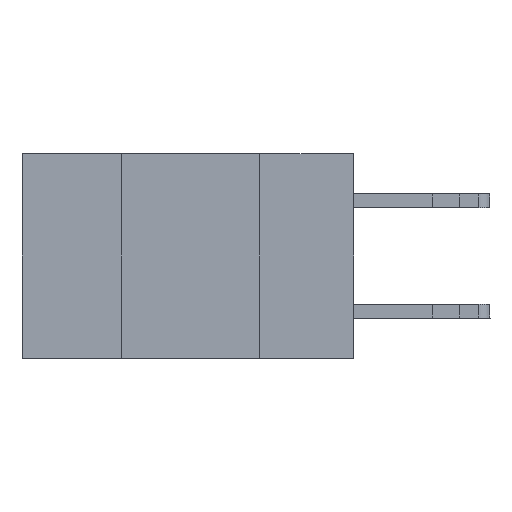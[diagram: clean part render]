
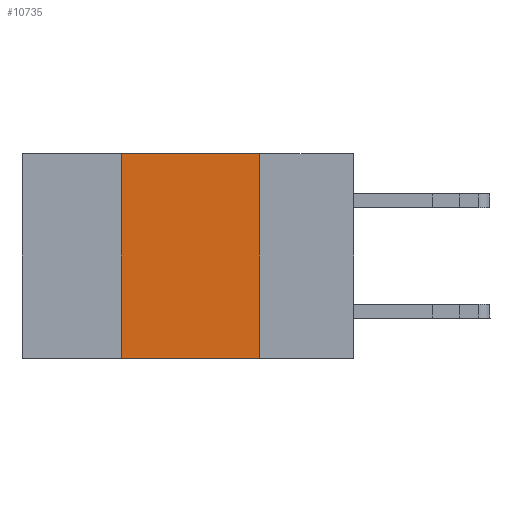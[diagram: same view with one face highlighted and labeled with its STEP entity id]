
A CAD part, left-side view. The second image highlights one B-rep face of the part: STEP entity #10735.
In plain terms, the highlighted planar face has unit normal (-1, 0, 0).
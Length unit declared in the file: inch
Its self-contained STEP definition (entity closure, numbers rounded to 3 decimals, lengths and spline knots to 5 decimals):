
#578 = EDGE_CURVE ( 'NONE', #19235, #1593, #18626, .T. ) ;
#873 = LINE ( 'NONE', #1668, #14500 ) ;
#1593 = VERTEX_POINT ( 'NONE', #20827 ) ;
#1668 = CARTESIAN_POINT ( 'NONE',  ( 0., 0.17, 0. ) ) ;
#1805 = FACE_OUTER_BOUND ( 'NONE', #4967, .T. ) ;
#2194 = DIRECTION ( 'NONE',  ( 0., -1., 0. ) ) ;
#3509 = LINE ( 'NONE', #20020, #16504 ) ;
#4251 = CARTESIAN_POINT ( 'NONE',  ( 0., 0.42, -0.37 ) ) ;
#4628 = DIRECTION ( 'NONE',  ( 0., 0., 1. ) ) ;
#4967 = EDGE_LOOP ( 'NONE', ( #20766, #8274, #18511, #7279 ) ) ;
#5052 = DIRECTION ( 'NONE',  ( 0., 0., -1. ) ) ;
#5714 = VECTOR ( 'NONE', #4628, 39.37008 ) ;
#7279 = ORIENTED_EDGE ( 'NONE', *, *, #16860, .T. ) ;
#8274 = ORIENTED_EDGE ( 'NONE', *, *, #10631, .F. ) ;
#8470 = DIRECTION ( 'NONE',  ( 0., 0., -1. ) ) ;
#9237 = CARTESIAN_POINT ( 'NONE',  ( 0., 0.6, 0. ) ) ;
#10277 = AXIS2_PLACEMENT_3D ( 'NONE', #9237, #15205, #5052 ) ;
#10631 = EDGE_CURVE ( 'NONE', #1593, #13225, #21349, .T. ) ;
#10735 = ADVANCED_FACE ( 'NONE', ( #1805 ), #17678, .F. ) ;
#11419 = CARTESIAN_POINT ( 'NONE',  ( 0., 0.17, -0.37 ) ) ;
#13225 = VERTEX_POINT ( 'NONE', #18328 ) ;
#14500 = VECTOR ( 'NONE', #8470, 39.37008 ) ;
#14962 = VERTEX_POINT ( 'NONE', #11419 ) ;
#15157 = DIRECTION ( 'NONE',  ( 0., -1., 0. ) ) ;
#15205 = DIRECTION ( 'NONE',  ( 1., 0., 0. ) ) ;
#16504 = VECTOR ( 'NONE', #15157, 39.37008 ) ;
#16860 = EDGE_CURVE ( 'NONE', #19235, #14962, #3509, .T. ) ;
#16963 = VECTOR ( 'NONE', #2194, 39.37008 ) ;
#17678 = PLANE ( 'NONE',  #10277 ) ;
#18328 = CARTESIAN_POINT ( 'NONE',  ( 0., 0.17, 0. ) ) ;
#18511 = ORIENTED_EDGE ( 'NONE', *, *, #578, .F. ) ;
#18626 = LINE ( 'NONE', #19802, #5714 ) ;
#19051 = CARTESIAN_POINT ( 'NONE',  ( 0., 0.6, 0. ) ) ;
#19235 = VERTEX_POINT ( 'NONE', #4251 ) ;
#19802 = CARTESIAN_POINT ( 'NONE',  ( 0., 0.42, 0. ) ) ;
#20020 = CARTESIAN_POINT ( 'NONE',  ( 0., 0.6, -0.37 ) ) ;
#20709 = EDGE_CURVE ( 'NONE', #13225, #14962, #873, .T. ) ;
#20766 = ORIENTED_EDGE ( 'NONE', *, *, #20709, .F. ) ;
#20827 = CARTESIAN_POINT ( 'NONE',  ( 0., 0.42, 0. ) ) ;
#21349 = LINE ( 'NONE', #19051, #16963 ) ;
